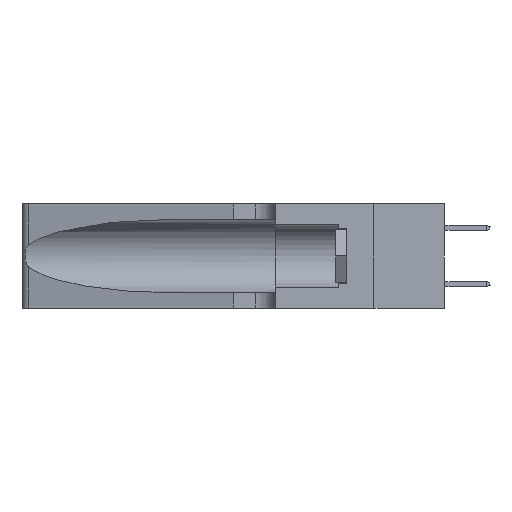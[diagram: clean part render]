
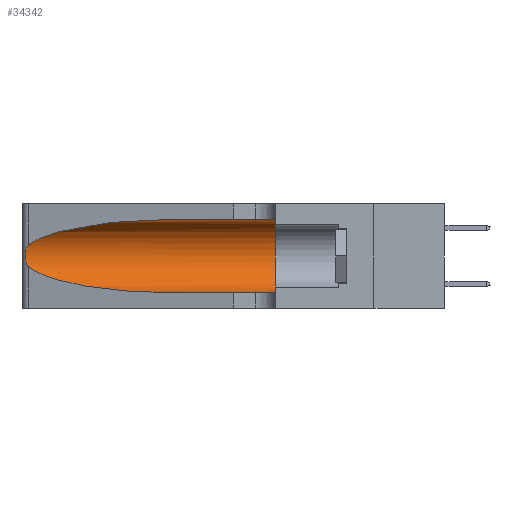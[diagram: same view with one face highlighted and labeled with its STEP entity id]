
A CAD part, left-side view. The second image highlights one B-rep face of the part: STEP entity #34342.
In plain terms, the highlighted cylindrical face has radius 3.308 mm (diameter 6.617 mm), a partial arc.
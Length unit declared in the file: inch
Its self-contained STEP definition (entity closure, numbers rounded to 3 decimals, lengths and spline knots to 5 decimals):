
#183 = CARTESIAN_POINT ( 'NONE',  ( 0.25639, 1.23184, 0.21858 ) ) ;
#357 = CARTESIAN_POINT ( 'NONE',  ( 0.26018, 1.23835, 0.19895 ) ) ;
#921 = CARTESIAN_POINT ( 'NONE',  ( 0.1305, 1.61858, 0.31525 ) ) ;
#1115 = AXIS2_PLACEMENT_3D ( 'NONE', #18275, #14398, #40131 ) ;
#2694 = EDGE_CURVE ( 'NONE', #40021, #9856, #20953, .T. ) ;
#5944 = FACE_OUTER_BOUND ( 'NONE', #21444, .T. ) ;
#6038 = DIRECTION ( 'NONE',  ( 0., -1., 0. ) ) ;
#8320 = LINE ( 'NONE', #921, #28110 ) ;
#9516 = VERTEX_POINT ( 'NONE', #17052 ) ;
#9856 = VERTEX_POINT ( 'NONE', #27106 ) ;
#10142 = CARTESIAN_POINT ( 'NONE',  ( 0.1305, 0.72297, 0.31525 ) ) ;
#10896 = ORIENTED_EDGE ( 'NONE', *, *, #24100, .F. ) ;
#10937 = CARTESIAN_POINT ( 'NONE',  ( 0.25487, 1.22718, 0.22369 ) ) ;
#11094 = CARTESIAN_POINT ( 'NONE',  ( 0.26075, 1.23896, 0.19203 ) ) ;
#11438 = CARTESIAN_POINT ( 'NONE',  ( 0.1305, 0.72297, 0.05475 ) ) ;
#11571 = CARTESIAN_POINT ( 'NONE',  ( 0.25856, 1.23593, 0.16098 ) ) ;
#13106 = EDGE_CURVE ( 'NONE', #18726, #9516, #32412, .T. ) ;
#13209 = ORIENTED_EDGE ( 'NONE', *, *, #15113, .T. ) ;
#13576 = CARTESIAN_POINT ( 'NONE',  ( 0.18966, 0.96281, 0.31525 ) ) ;
#14398 = DIRECTION ( 'NONE',  ( 0., -1., 0. ) ) ;
#14462 = CARTESIAN_POINT ( 'NONE',  ( 0.25487, 1.22718, 0.14631 ) ) ;
#14674 = CARTESIAN_POINT ( 'NONE',  ( 0.25854, 1.2359, 0.20912 ) ) ;
#15085 =( BOUNDED_CURVE ( )  B_SPLINE_CURVE ( 3, ( #10142, #13576, #39604, #17307 ),
 .UNSPECIFIED., .F., .T. ) 
 B_SPLINE_CURVE_WITH_KNOTS ( ( 4, 4 ),
 ( 1.5708, 2.84003 ),
 .UNSPECIFIED. ) 
 CURVE ( )  GEOMETRIC_REPRESENTATION_ITEM ( )  RATIONAL_B_SPLINE_CURVE ( ( 1., 0.87, 0.87, 1. ) ) 
 REPRESENTATION_ITEM ( '' )  );
#15113 = EDGE_CURVE ( 'NONE', #26056, #18726, #15085, .T. ) ;
#15359 = CARTESIAN_POINT ( 'NONE',  ( 0.1305, 0.35, 0.31525 ) ) ;
#15883 = DIRECTION ( 'NONE',  ( 0., 0., 1. ) ) ;
#16378 = CARTESIAN_POINT ( 'NONE',  ( 0.1305, 0.35, 0.185 ) ) ;
#17052 = CARTESIAN_POINT ( 'NONE',  ( 0.25487, 1.22718, 0.14631 ) ) ;
#17307 = CARTESIAN_POINT ( 'NONE',  ( 0.25487, 1.22718, 0.22369 ) ) ;
#17898 = EDGE_CURVE ( 'NONE', #9516, #28434, #43181, .T. ) ;
#18275 = CARTESIAN_POINT ( 'NONE',  ( 0.1305, 1.61858, 0.185 ) ) ;
#18403 = CARTESIAN_POINT ( 'NONE',  ( 0.25639, 1.23186, 0.15144 ) ) ;
#18726 = VERTEX_POINT ( 'NONE', #28686 ) ;
#19377 = ORIENTED_EDGE ( 'NONE', *, *, #22879, .T. ) ;
#20953 = CIRCLE ( 'NONE', #47451, 0.13025 ) ;
#21444 = EDGE_LOOP ( 'NONE', ( #13209, #47151, #21706, #19377, #30064, #10896 ) ) ;
#21706 = ORIENTED_EDGE ( 'NONE', *, *, #17898, .T. ) ;
#21902 = CARTESIAN_POINT ( 'NONE',  ( 0.18966, 0.96281, 0.05475 ) ) ;
#22125 = CARTESIAN_POINT ( 'NONE',  ( 0.25487, 1.22718, 0.14631 ) ) ;
#22617 = CARTESIAN_POINT ( 'NONE',  ( 0.25787, 1.23484, 0.2124 ) ) ;
#22879 = EDGE_CURVE ( 'NONE', #28434, #9856, #32305, .T. ) ;
#23210 = DIRECTION ( 'NONE',  ( 0., 1., 0. ) ) ;
#24100 = EDGE_CURVE ( 'NONE', #26056, #40021, #8320, .T. ) ;
#25527 = CARTESIAN_POINT ( 'NONE',  ( 0.2373, 1.15595, 0.08982 ) ) ;
#26056 = VERTEX_POINT ( 'NONE', #47508 ) ;
#26060 = CARTESIAN_POINT ( 'NONE',  ( 0.26017, 1.23833, 0.17102 ) ) ;
#27106 = CARTESIAN_POINT ( 'NONE',  ( 0.1305, 0.35, 0.05475 ) ) ;
#28110 = VECTOR ( 'NONE', #30663, 39.37008 ) ;
#28434 = VERTEX_POINT ( 'NONE', #11438 ) ;
#28686 = CARTESIAN_POINT ( 'NONE',  ( 0.25487, 1.22718, 0.22369 ) ) ;
#30064 = ORIENTED_EDGE ( 'NONE', *, *, #2694, .F. ) ;
#30663 = DIRECTION ( 'NONE',  ( 0., -1., 0. ) ) ;
#32305 = LINE ( 'NONE', #38902, #39871 ) ;
#32412 = B_SPLINE_CURVE_WITH_KNOTS ( 'NONE', 3,
 ( #10937, #37463, #183, #22617, #14674, #357, #11094, #33870, #26060, #11571, #40730, #18403, #44457, #22125 ),
 .UNSPECIFIED., .F., .F.,
 ( 4, 2, 2, 2, 2, 2, 4 ),
 ( 0., 0.00027, 0.00053, 0.00107, 0.0016, 0.00187, 0.00214 ),
 .UNSPECIFIED. ) ;
#32691 = CARTESIAN_POINT ( 'NONE',  ( 0.1305, 0.72297, 0.05475 ) ) ;
#33870 = CARTESIAN_POINT ( 'NONE',  ( 0.26075, 1.23896, 0.178 ) ) ;
#34342 = ADVANCED_FACE ( 'NONE', ( #5944 ), #44899, .F. ) ;
#37463 = CARTESIAN_POINT ( 'NONE',  ( 0.25555, 1.22994, 0.2215 ) ) ;
#38902 = CARTESIAN_POINT ( 'NONE',  ( 0.1305, 1.61858, 0.05475 ) ) ;
#39604 = CARTESIAN_POINT ( 'NONE',  ( 0.2373, 1.15595, 0.28018 ) ) ;
#39871 = VECTOR ( 'NONE', #6038, 39.37008 ) ;
#40021 = VERTEX_POINT ( 'NONE', #15359 ) ;
#40131 = DIRECTION ( 'NONE',  ( 0., 0., -1. ) ) ;
#40730 = CARTESIAN_POINT ( 'NONE',  ( 0.25789, 1.23486, 0.15765 ) ) ;
#43181 =( BOUNDED_CURVE ( )  B_SPLINE_CURVE ( 3, ( #14462, #25527, #21902, #32691 ),
 .UNSPECIFIED., .F., .F. ) 
 B_SPLINE_CURVE_WITH_KNOTS ( ( 4, 4 ),
 ( 3.44316, 4.71239 ),
 .UNSPECIFIED. ) 
 CURVE ( )  GEOMETRIC_REPRESENTATION_ITEM ( )  RATIONAL_B_SPLINE_CURVE ( ( 1., 0.87, 0.87, 1. ) ) 
 REPRESENTATION_ITEM ( '' )  );
#44457 = CARTESIAN_POINT ( 'NONE',  ( 0.25555, 1.22993, 0.14849 ) ) ;
#44899 = CYLINDRICAL_SURFACE ( 'NONE', #1115, 0.13025 ) ;
#47151 = ORIENTED_EDGE ( 'NONE', *, *, #13106, .T. ) ;
#47451 = AXIS2_PLACEMENT_3D ( 'NONE', #16378, #23210, #15883 ) ;
#47508 = CARTESIAN_POINT ( 'NONE',  ( 0.1305, 0.72297, 0.31525 ) ) ;
